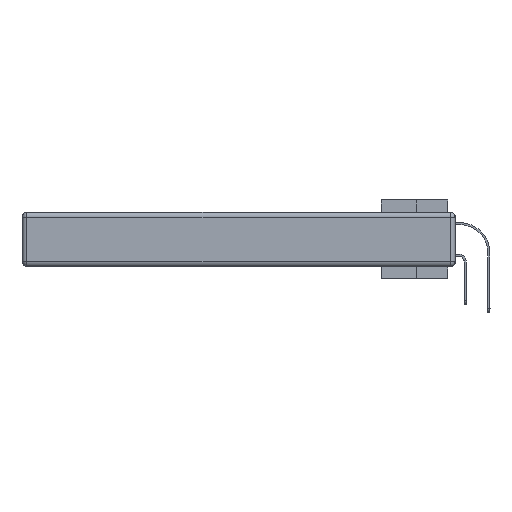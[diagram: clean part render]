
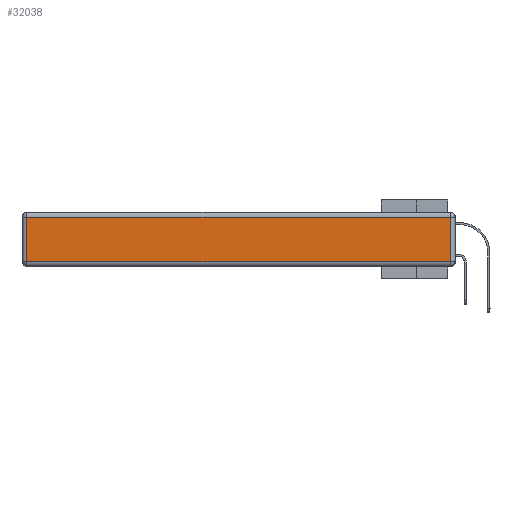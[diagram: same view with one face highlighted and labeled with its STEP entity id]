
A CAD part, left-side view. The second image highlights one B-rep face of the part: STEP entity #32038.
In plain terms, the highlighted planar face has unit normal (-1, 0, 0).
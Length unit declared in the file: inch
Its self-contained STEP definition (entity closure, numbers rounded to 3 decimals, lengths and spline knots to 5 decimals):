
#543 = DIRECTION ( 'NONE',  ( 0., -1., 0. ) ) ;
#3020 = PLANE ( 'NONE',  #33155 ) ;
#3080 = CARTESIAN_POINT ( 'NONE',  ( 0., 0.03, -0.343 ) ) ;
#4718 = ORIENTED_EDGE ( 'NONE', *, *, #7762, .T. ) ;
#7762 = EDGE_CURVE ( 'NONE', #33420, #34808, #22122, .T. ) ;
#8065 = VERTEX_POINT ( 'NONE', #34044 ) ;
#9663 = CARTESIAN_POINT ( 'NONE',  ( 0., 2.75, -0.03 ) ) ;
#9908 = DIRECTION ( 'NONE',  ( 0., 0., 1. ) ) ;
#12758 = DIRECTION ( 'NONE',  ( 0., 0., 1. ) ) ;
#13185 = VERTEX_POINT ( 'NONE', #33575 ) ;
#15829 = LINE ( 'NONE', #16666, #37685 ) ;
#15999 = EDGE_CURVE ( 'NONE', #34808, #13185, #25405, .T. ) ;
#16666 = CARTESIAN_POINT ( 'NONE',  ( 0., 0., -0.313 ) ) ;
#17114 = VECTOR ( 'NONE', #33038, 39.37008 ) ;
#17690 = ORIENTED_EDGE ( 'NONE', *, *, #22424, .T. ) ;
#18743 = VECTOR ( 'NONE', #22289, 39.37008 ) ;
#21327 = ORIENTED_EDGE ( 'NONE', *, *, #30751, .T. ) ;
#22122 = LINE ( 'NONE', #3080, #34390 ) ;
#22289 = DIRECTION ( 'NONE',  ( 0., 1., 0. ) ) ;
#22424 = EDGE_CURVE ( 'NONE', #13185, #8065, #33437, .T. ) ;
#25405 = LINE ( 'NONE', #9663, #18743 ) ;
#25566 = DIRECTION ( 'NONE',  ( -1., 0., 0. ) ) ;
#28671 = CARTESIAN_POINT ( 'NONE',  ( 0., 0., -0.343 ) ) ;
#29773 = CARTESIAN_POINT ( 'NONE',  ( 0., 2.72, -0.343 ) ) ;
#30751 = EDGE_CURVE ( 'NONE', #8065, #33420, #15829, .T. ) ;
#31464 = CARTESIAN_POINT ( 'NONE',  ( 0., 0.03, -0.03 ) ) ;
#32038 = ADVANCED_FACE ( 'NONE', ( #33482 ), #3020, .T. ) ;
#33038 = DIRECTION ( 'NONE',  ( 0., 0., -1. ) ) ;
#33155 = AXIS2_PLACEMENT_3D ( 'NONE', #28671, #25566, #12758 ) ;
#33420 = VERTEX_POINT ( 'NONE', #37949 ) ;
#33437 = LINE ( 'NONE', #29773, #17114 ) ;
#33482 = FACE_OUTER_BOUND ( 'NONE', #37973, .T. ) ;
#33575 = CARTESIAN_POINT ( 'NONE',  ( 0., 2.72, -0.03 ) ) ;
#34044 = CARTESIAN_POINT ( 'NONE',  ( 0., 2.72, -0.313 ) ) ;
#34390 = VECTOR ( 'NONE', #9908, 39.37008 ) ;
#34808 = VERTEX_POINT ( 'NONE', #31464 ) ;
#37685 = VECTOR ( 'NONE', #543, 39.37008 ) ;
#37949 = CARTESIAN_POINT ( 'NONE',  ( 0., 0.03, -0.313 ) ) ;
#37973 = EDGE_LOOP ( 'NONE', ( #21327, #4718, #40079, #17690 ) ) ;
#40079 = ORIENTED_EDGE ( 'NONE', *, *, #15999, .T. ) ;
